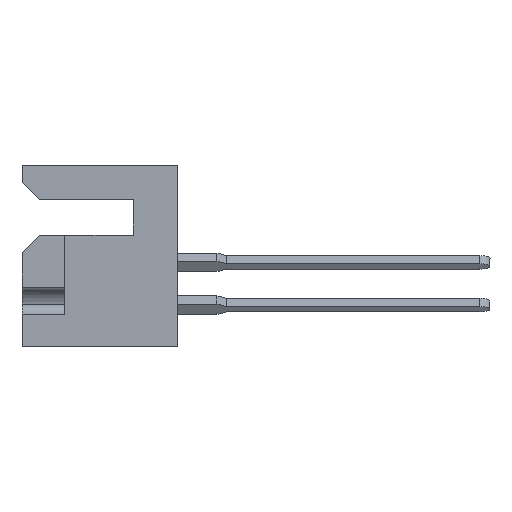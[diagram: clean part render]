
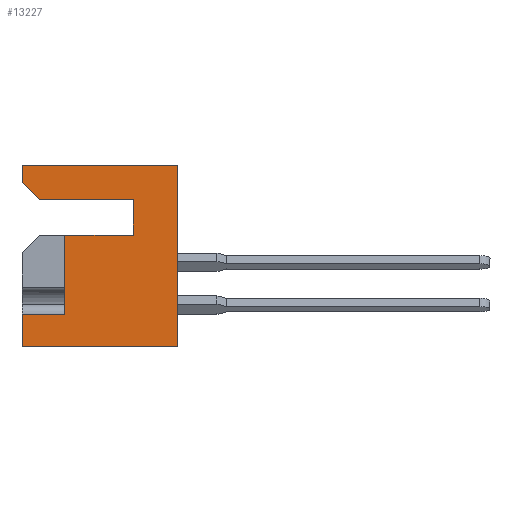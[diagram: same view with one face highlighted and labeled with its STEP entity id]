
A CAD part, left-side view. The second image highlights one B-rep face of the part: STEP entity #13227.
In plain terms, the highlighted planar face has unit normal (-1, 0, 0).
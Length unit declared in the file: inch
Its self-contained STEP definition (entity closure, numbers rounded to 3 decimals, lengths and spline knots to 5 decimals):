
#13 = ORIENTED_EDGE ( 'NONE', *, *, #4177, .F. ) ;
#180 = LINE ( 'NONE', #10797, #7518 ) ;
#190 = CARTESIAN_POINT ( 'NONE',  ( 0., 0.128, -0.205 ) ) ;
#728 = CARTESIAN_POINT ( 'NONE',  ( 0., 0.453, 0. ) ) ;
#921 = CARTESIAN_POINT ( 'NONE',  ( 0., 0., -0.531 ) ) ;
#1136 = EDGE_LOOP ( 'NONE', ( #2751, #15131, #5686, #11483, #13, #12849, #15863, #8556, #10193, #16056, #16377 ) ) ;
#1159 = EDGE_CURVE ( 'NONE', #1681, #9903, #9581, .T. ) ;
#1546 = CARTESIAN_POINT ( 'NONE',  ( 0., 0.128, -0.1 ) ) ;
#1681 = VERTEX_POINT ( 'NONE', #12399 ) ;
#1877 = DIRECTION ( 'NONE',  ( 0., 0., 1. ) ) ;
#1928 = DIRECTION ( 'NONE',  ( 0., 0., 1. ) ) ;
#2287 = LINE ( 'NONE', #5988, #2681 ) ;
#2420 = DIRECTION ( 'NONE',  ( 0., 1., 0. ) ) ;
#2581 = CARTESIAN_POINT ( 'NONE',  ( 0., 0.453, 0. ) ) ;
#2618 = VERTEX_POINT ( 'NONE', #9562 ) ;
#2681 = VECTOR ( 'NONE', #7383, 39.37008 ) ;
#2748 = DIRECTION ( 'NONE',  ( 0., 1., 0. ) ) ;
#2751 = ORIENTED_EDGE ( 'NONE', *, *, #1159, .T. ) ;
#2967 = VERTEX_POINT ( 'NONE', #6471 ) ;
#3078 = VERTEX_POINT ( 'NONE', #12972 ) ;
#3119 = FACE_OUTER_BOUND ( 'NONE', #1136, .T. ) ;
#3226 = DIRECTION ( 'NONE',  ( 0., 0., 1. ) ) ;
#3260 = EDGE_CURVE ( 'NONE', #14824, #3535, #14416, .T. ) ;
#3535 = VERTEX_POINT ( 'NONE', #2581 ) ;
#3866 = LINE ( 'NONE', #1546, #4053 ) ;
#4053 = VECTOR ( 'NONE', #11691, 39.37008 ) ;
#4149 = LINE ( 'NONE', #6174, #11694 ) ;
#4156 = CARTESIAN_POINT ( 'NONE',  ( 0., 0.453, -0.531 ) ) ;
#4177 = EDGE_CURVE ( 'NONE', #3535, #2967, #10632, .T. ) ;
#4183 = VECTOR ( 'NONE', #2748, 39.37008 ) ;
#4409 = DIRECTION ( 'NONE',  ( 0., -1., 0. ) ) ;
#4539 = VECTOR ( 'NONE', #5627, 39.37008 ) ;
#4897 = CARTESIAN_POINT ( 'NONE',  ( 0., 0.328, -0.437 ) ) ;
#4933 = LINE ( 'NONE', #4156, #4539 ) ;
#4945 = EDGE_CURVE ( 'NONE', #1681, #13183, #2287, .T. ) ;
#4969 = LINE ( 'NONE', #190, #4183 ) ;
#5627 = DIRECTION ( 'NONE',  ( 0., -1., 0. ) ) ;
#5686 = ORIENTED_EDGE ( 'NONE', *, *, #10786, .T. ) ;
#5757 = CARTESIAN_POINT ( 'NONE',  ( 0., 0.328, -0.205 ) ) ;
#5962 = EDGE_CURVE ( 'NONE', #14824, #2618, #8559, .T. ) ;
#5977 = DIRECTION ( 'NONE',  ( 0., 0., -1. ) ) ;
#5988 = CARTESIAN_POINT ( 'NONE',  ( 0., 0.328, -0.205 ) ) ;
#6035 = CARTESIAN_POINT ( 'NONE',  ( 0., 0.453, 0. ) ) ;
#6149 = PLANE ( 'NONE',  #6357 ) ;
#6174 = CARTESIAN_POINT ( 'NONE',  ( 0., 0., 0. ) ) ;
#6357 = AXIS2_PLACEMENT_3D ( 'NONE', #6035, #12326, #5977 ) ;
#6471 = CARTESIAN_POINT ( 'NONE',  ( 0., 0., 0. ) ) ;
#7085 = EDGE_CURVE ( 'NONE', #16027, #13183, #4969, .T. ) ;
#7383 = DIRECTION ( 'NONE',  ( 0., 0., 1. ) ) ;
#7462 = EDGE_CURVE ( 'NONE', #3078, #9903, #13103, .T. ) ;
#7518 = VECTOR ( 'NONE', #1877, 39.37008 ) ;
#7803 = VERTEX_POINT ( 'NONE', #15442 ) ;
#7893 = VECTOR ( 'NONE', #1928, 39.37008 ) ;
#8556 = ORIENTED_EDGE ( 'NONE', *, *, #15661, .F. ) ;
#8559 = LINE ( 'NONE', #9346, #10361 ) ;
#8920 = VECTOR ( 'NONE', #3226, 39.37008 ) ;
#9236 = VECTOR ( 'NONE', #4409, 39.37008 ) ;
#9346 = CARTESIAN_POINT ( 'NONE',  ( 0., 0.403, -0.1 ) ) ;
#9370 = CARTESIAN_POINT ( 'NONE',  ( 0., 0.453, -0.05 ) ) ;
#9494 = CARTESIAN_POINT ( 'NONE',  ( 0., 0.453, 0. ) ) ;
#9562 = CARTESIAN_POINT ( 'NONE',  ( 0., 0.403, -0.1 ) ) ;
#9581 = LINE ( 'NONE', #4897, #12194 ) ;
#9903 = VERTEX_POINT ( 'NONE', #16284 ) ;
#10193 = ORIENTED_EDGE ( 'NONE', *, *, #10935, .F. ) ;
#10361 = VECTOR ( 'NONE', #10647, 39.37008 ) ;
#10632 = LINE ( 'NONE', #14500, #9236 ) ;
#10647 = DIRECTION ( 'NONE',  ( 0., -0.707, -0.707 ) ) ;
#10786 = EDGE_CURVE ( 'NONE', #3078, #12626, #4933, .T. ) ;
#10797 = CARTESIAN_POINT ( 'NONE',  ( 0., 0.128, -0.1 ) ) ;
#10935 = EDGE_CURVE ( 'NONE', #16027, #7803, #180, .T. ) ;
#10990 = EDGE_CURVE ( 'NONE', #12626, #2967, #4149, .T. ) ;
#11483 = ORIENTED_EDGE ( 'NONE', *, *, #10990, .T. ) ;
#11691 = DIRECTION ( 'NONE',  ( 0., 1., 0. ) ) ;
#11694 = VECTOR ( 'NONE', #16196, 39.37008 ) ;
#12194 = VECTOR ( 'NONE', #2420, 39.37008 ) ;
#12326 = DIRECTION ( 'NONE',  ( 1., 0., 0. ) ) ;
#12399 = CARTESIAN_POINT ( 'NONE',  ( 0., 0.328, -0.437 ) ) ;
#12626 = VERTEX_POINT ( 'NONE', #921 ) ;
#12849 = ORIENTED_EDGE ( 'NONE', *, *, #3260, .F. ) ;
#12972 = CARTESIAN_POINT ( 'NONE',  ( 0., 0.453, -0.531 ) ) ;
#13103 = LINE ( 'NONE', #728, #8920 ) ;
#13183 = VERTEX_POINT ( 'NONE', #5757 ) ;
#13227 = ADVANCED_FACE ( 'NONE', ( #3119 ), #6149, .F. ) ;
#14416 = LINE ( 'NONE', #9494, #7893 ) ;
#14500 = CARTESIAN_POINT ( 'NONE',  ( 0., 0.453, 0. ) ) ;
#14750 = CARTESIAN_POINT ( 'NONE',  ( 0., 0.128, -0.205 ) ) ;
#14824 = VERTEX_POINT ( 'NONE', #9370 ) ;
#15131 = ORIENTED_EDGE ( 'NONE', *, *, #7462, .F. ) ;
#15442 = CARTESIAN_POINT ( 'NONE',  ( 0., 0.128, -0.1 ) ) ;
#15661 = EDGE_CURVE ( 'NONE', #7803, #2618, #3866, .T. ) ;
#15863 = ORIENTED_EDGE ( 'NONE', *, *, #5962, .T. ) ;
#16027 = VERTEX_POINT ( 'NONE', #14750 ) ;
#16056 = ORIENTED_EDGE ( 'NONE', *, *, #7085, .T. ) ;
#16196 = DIRECTION ( 'NONE',  ( 0., 0., 1. ) ) ;
#16284 = CARTESIAN_POINT ( 'NONE',  ( 0., 0.453, -0.437 ) ) ;
#16377 = ORIENTED_EDGE ( 'NONE', *, *, #4945, .F. ) ;
